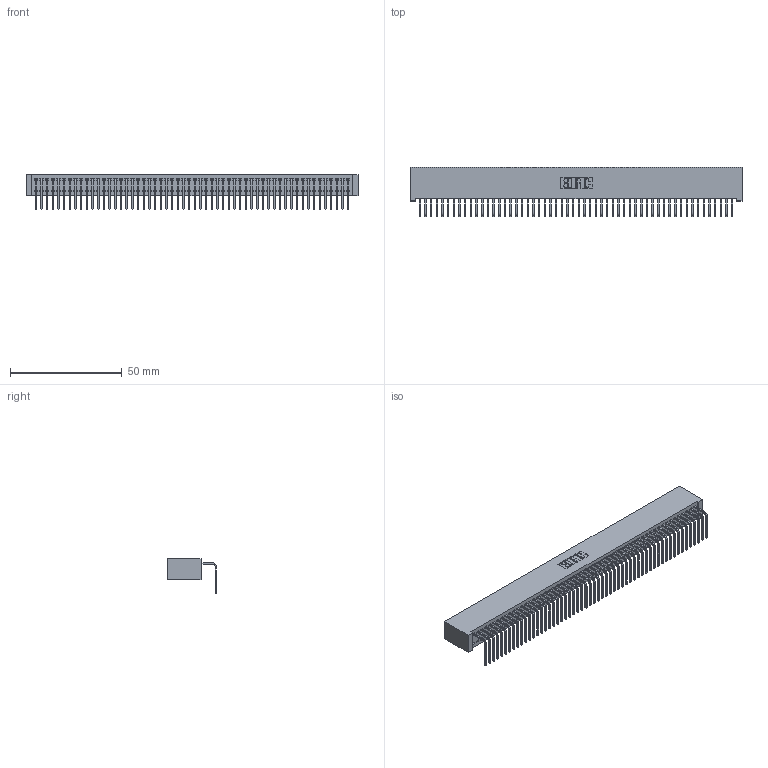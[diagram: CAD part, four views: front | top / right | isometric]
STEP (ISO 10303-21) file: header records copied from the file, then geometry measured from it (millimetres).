
FILE_DESCRIPTION (( 'STEP AP203' ), '1' );
FILE_NAME ('342-056-558-101.STEP', '2019-10-03T11:40:47', ( '' ), ( '' ), 'SwSTEP 2.0', 'SolidWorks 2016', '' );
FILE_SCHEMA (( 'CONFIG_CONTROL_DESIGN' ));
Length unit declared in the file: inch
Products named in the file (3): 345-292-001_558 Tail - 2; 342-056-558-101; 342 Part_Lugless
Assembly tree (57 placements, depth 2):
  342-056-558-101
    342 Part_Lugless
    345-292-001_558 Tail - 2  x56
Bounding box: 148.49 x 21.91 x 15.62 mm (x, y, z)
Volume: 13666.6 mm3; surface area: 21713.1 mm2
Topology: 57 solids, 57 shells, 3462 faces, 10467 edges, 6902 vertices
Faces by surface type: plane 2526, cylinder 936
Entity records: 32099 total; most frequent: CARTESIAN_POINT 5542, ORIENTED_EDGE 5534, DIRECTION 4639, EDGE_CURVE 2767, VECTOR 2647, LINE 2647, VERTEX_POINT 1842, AXIS2_PLACEMENT_3D 996
